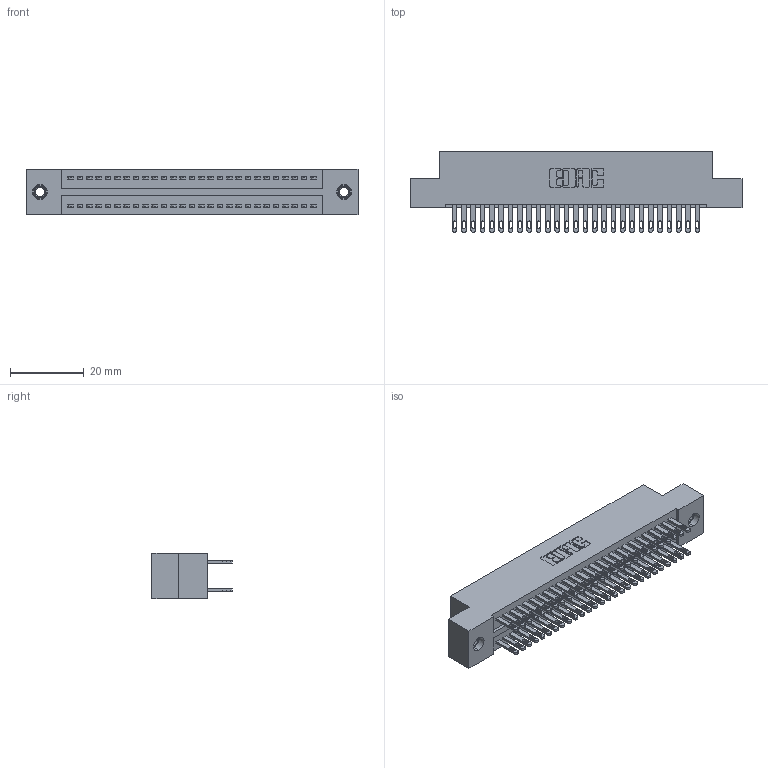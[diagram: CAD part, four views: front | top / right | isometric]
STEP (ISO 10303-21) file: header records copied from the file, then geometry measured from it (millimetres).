
FILE_DESCRIPTION (( 'STEP AP203' ), '1' );
FILE_NAME ('325-054-500-207.STEP', '2020-02-25T00:49:57', ( '' ), ( '' ), 'SwSTEP 2.0', 'SolidWorks 2016', '' );
FILE_SCHEMA (( 'CONFIG_CONTROL_DESIGN' ));
Length unit declared in the file: inch
Products named in the file (4): 325 Part_TI; 345-250-001_345-250-005-103; 325-054-500-207; 325-292-001_325-293-100
Assembly tree (57 placements, depth 2):
  325-054-500-207
    325 Part_TI
    325-292-001_325-293-100  x54
    345-250-001_345-250-005-103  x2
Bounding box: 90.3 x 21.84 x 12.45 mm (x, y, z)
Volume: 11673.8 mm3; surface area: 14364.8 mm2
Topology: 57 solids, 57 shells, 2766 faces, 8385 edges, 5582 vertices
Faces by surface type: plane 1722, cylinder 1028, cone 12, torus 4
Entity records: 20426 total; most frequent: CARTESIAN_POINT 3385, ORIENTED_EDGE 3314, DIRECTION 2951, EDGE_CURVE 1657, VECTOR 1505, LINE 1505, VERTEX_POINT 1100, AXIS2_PLACEMENT_3D 723
